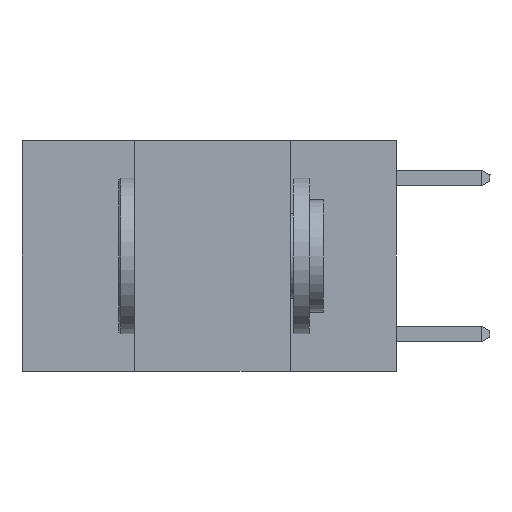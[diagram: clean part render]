
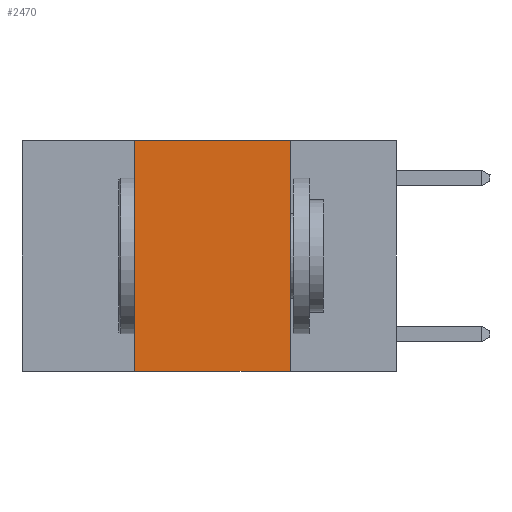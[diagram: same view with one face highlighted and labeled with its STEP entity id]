
A CAD part, left-side view. The second image highlights one B-rep face of the part: STEP entity #2470.
In plain terms, the highlighted planar face has unit normal (-1, 0, 0).
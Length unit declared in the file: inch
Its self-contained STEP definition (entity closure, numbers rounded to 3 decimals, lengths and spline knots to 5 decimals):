
#355 = PLANE ( 'NONE',  #689 ) ;
#689 = AXIS2_PLACEMENT_3D ( 'NONE', #9512, #4342, #10350 ) ;
#746 = VERTEX_POINT ( 'NONE', #822 ) ;
#822 = CARTESIAN_POINT ( 'NONE',  ( 0., 0.17, 0. ) ) ;
#938 = DIRECTION ( 'NONE',  ( 0., -1., 0. ) ) ;
#972 = DIRECTION ( 'NONE',  ( 0., 0., 1. ) ) ;
#1261 = LINE ( 'NONE', #5689, #1897 ) ;
#1655 = VERTEX_POINT ( 'NONE', #7475 ) ;
#1897 = VECTOR ( 'NONE', #972, 39.37008 ) ;
#1960 = CARTESIAN_POINT ( 'NONE',  ( 0., 0.17, -0.37 ) ) ;
#2053 = VERTEX_POINT ( 'NONE', #1960 ) ;
#2155 = LINE ( 'NONE', #4178, #11167 ) ;
#2355 = VECTOR ( 'NONE', #10028, 39.37008 ) ;
#2410 = CARTESIAN_POINT ( 'NONE',  ( 0., 0.42, 0. ) ) ;
#2470 = ADVANCED_FACE ( 'NONE', ( #3149 ), #355, .F. ) ;
#3149 = FACE_OUTER_BOUND ( 'NONE', #4899, .T. ) ;
#3806 = LINE ( 'NONE', #9884, #10444 ) ;
#4178 = CARTESIAN_POINT ( 'NONE',  ( 0., 0.6, -0.37 ) ) ;
#4342 = DIRECTION ( 'NONE',  ( 1., 0., 0. ) ) ;
#4353 = ORIENTED_EDGE ( 'NONE', *, *, #5661, .F. ) ;
#4899 = EDGE_LOOP ( 'NONE', ( #4353, #10998, #11389, #10837 ) ) ;
#5134 = LINE ( 'NONE', #8336, #2355 ) ;
#5535 = EDGE_CURVE ( 'NONE', #9299, #746, #3806, .T. ) ;
#5661 = EDGE_CURVE ( 'NONE', #746, #2053, #5134, .T. ) ;
#5689 = CARTESIAN_POINT ( 'NONE',  ( 0., 0.42, 0. ) ) ;
#6011 = DIRECTION ( 'NONE',  ( 0., -1., 0. ) ) ;
#6278 = EDGE_CURVE ( 'NONE', #1655, #9299, #1261, .T. ) ;
#7475 = CARTESIAN_POINT ( 'NONE',  ( 0., 0.42, -0.37 ) ) ;
#8336 = CARTESIAN_POINT ( 'NONE',  ( 0., 0.17, 0. ) ) ;
#8533 = EDGE_CURVE ( 'NONE', #1655, #2053, #2155, .T. ) ;
#9299 = VERTEX_POINT ( 'NONE', #2410 ) ;
#9512 = CARTESIAN_POINT ( 'NONE',  ( 0., 0.6, 0. ) ) ;
#9884 = CARTESIAN_POINT ( 'NONE',  ( 0., 0.6, 0. ) ) ;
#10028 = DIRECTION ( 'NONE',  ( 0., 0., -1. ) ) ;
#10350 = DIRECTION ( 'NONE',  ( 0., 0., -1. ) ) ;
#10444 = VECTOR ( 'NONE', #938, 39.37008 ) ;
#10837 = ORIENTED_EDGE ( 'NONE', *, *, #8533, .T. ) ;
#10998 = ORIENTED_EDGE ( 'NONE', *, *, #5535, .F. ) ;
#11167 = VECTOR ( 'NONE', #6011, 39.37008 ) ;
#11389 = ORIENTED_EDGE ( 'NONE', *, *, #6278, .F. ) ;
